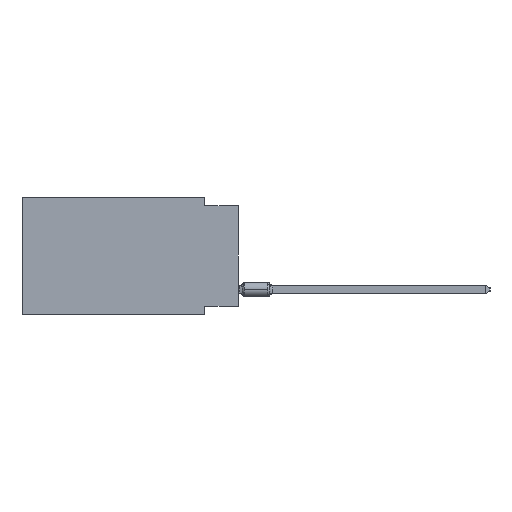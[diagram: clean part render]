
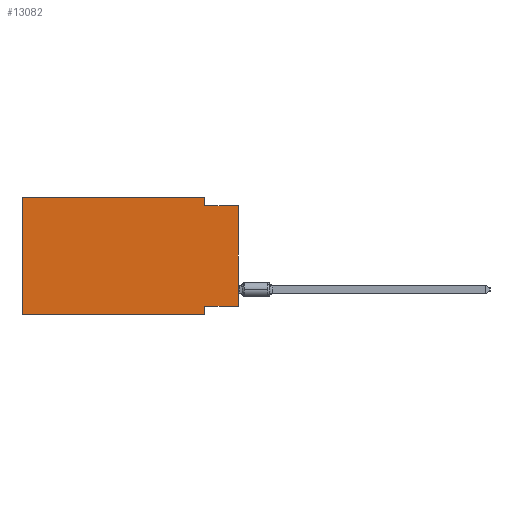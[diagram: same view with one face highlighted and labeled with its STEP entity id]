
A CAD part, left-side view. The second image highlights one B-rep face of the part: STEP entity #13082.
In plain terms, the highlighted planar face has unit normal (-1, 0, 0).
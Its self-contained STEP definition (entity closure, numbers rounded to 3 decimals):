
#56 = CARTESIAN_POINT ( 'NONE',  ( 0., 16.383, 0. ) ) ;
#1926 = LINE ( 'NONE', #31719, #31229 ) ;
#2910 = AXIS2_PLACEMENT_3D ( 'NONE', #56, #14715, #25537 ) ;
#2994 = VERTEX_POINT ( 'NONE', #15073 ) ;
#4694 = EDGE_LOOP ( 'NONE', ( #25086, #36051, #12913, #10213, #41114, #26272, #20955, #39437 ) ) ;
#7222 = VERTEX_POINT ( 'NONE', #24212 ) ;
#7512 = LINE ( 'NONE', #10891, #12361 ) ;
#8205 = VERTEX_POINT ( 'NONE', #41832 ) ;
#8336 = DIRECTION ( 'NONE',  ( 0., 0., -1. ) ) ;
#9957 = VERTEX_POINT ( 'NONE', #23891 ) ;
#10213 = ORIENTED_EDGE ( 'NONE', *, *, #20661, .F. ) ;
#10457 = VERTEX_POINT ( 'NONE', #16375 ) ;
#10891 = CARTESIAN_POINT ( 'NONE',  ( 0., 2.54, 0. ) ) ;
#11546 = EDGE_CURVE ( 'NONE', #20242, #8205, #12090, .T. ) ;
#12041 = EDGE_CURVE ( 'NONE', #31411, #2994, #1926, .T. ) ;
#12090 = LINE ( 'NONE', #23152, #43458 ) ;
#12361 = VECTOR ( 'NONE', #33438, 1000. ) ;
#12913 = ORIENTED_EDGE ( 'NONE', *, *, #18603, .F. ) ;
#13082 = ADVANCED_FACE ( 'NONE', ( #22160 ), #25290, .F. ) ;
#13092 = EDGE_CURVE ( 'NONE', #31411, #15208, #18311, .T. ) ;
#14375 = DIRECTION ( 'NONE',  ( 0., -1., 0. ) ) ;
#14715 = DIRECTION ( 'NONE',  ( 1., 0., 0. ) ) ;
#15073 = CARTESIAN_POINT ( 'NONE',  ( 0., 2.54, -8.89 ) ) ;
#15124 = VECTOR ( 'NONE', #8336, 1000. ) ;
#15208 = VERTEX_POINT ( 'NONE', #45181 ) ;
#16375 = CARTESIAN_POINT ( 'NONE',  ( 0., 2.54, -0.635 ) ) ;
#16580 = DIRECTION ( 'NONE',  ( 0., -1., 0. ) ) ;
#16876 = VECTOR ( 'NONE', #34235, 1000. ) ;
#17485 = EDGE_CURVE ( 'NONE', #10457, #8205, #45370, .T. ) ;
#18311 = LINE ( 'NONE', #22400, #28280 ) ;
#18560 = DIRECTION ( 'NONE',  ( 0., 0., 1. ) ) ;
#18603 = EDGE_CURVE ( 'NONE', #9957, #10457, #7512, .T. ) ;
#20021 = DIRECTION ( 'NONE',  ( 0., 0., 1. ) ) ;
#20242 = VERTEX_POINT ( 'NONE', #43735 ) ;
#20661 = EDGE_CURVE ( 'NONE', #15208, #9957, #37343, .T. ) ;
#20955 = ORIENTED_EDGE ( 'NONE', *, *, #42062, .F. ) ;
#22160 = FACE_OUTER_BOUND ( 'NONE', #4694, .T. ) ;
#22400 = CARTESIAN_POINT ( 'NONE',  ( 0., 16.383, 0. ) ) ;
#23152 = CARTESIAN_POINT ( 'NONE',  ( 0., 0., 0. ) ) ;
#23510 = DIRECTION ( 'NONE',  ( 0., -1., 0. ) ) ;
#23891 = CARTESIAN_POINT ( 'NONE',  ( 0., 2.54, 0. ) ) ;
#24212 = CARTESIAN_POINT ( 'NONE',  ( 0., 2.54, -8.255 ) ) ;
#25086 = ORIENTED_EDGE ( 'NONE', *, *, #11546, .T. ) ;
#25290 = PLANE ( 'NONE',  #2910 ) ;
#25537 = DIRECTION ( 'NONE',  ( 0., 0., -1. ) ) ;
#26272 = ORIENTED_EDGE ( 'NONE', *, *, #12041, .T. ) ;
#26970 = VECTOR ( 'NONE', #14375, 1000. ) ;
#27768 = LINE ( 'NONE', #45751, #16876 ) ;
#28280 = VECTOR ( 'NONE', #18560, 1000. ) ;
#31229 = VECTOR ( 'NONE', #16580, 1000. ) ;
#31411 = VERTEX_POINT ( 'NONE', #39261 ) ;
#31719 = CARTESIAN_POINT ( 'NONE',  ( 0., 16.383, -8.89 ) ) ;
#33438 = DIRECTION ( 'NONE',  ( 0., 0., -1. ) ) ;
#33743 = EDGE_CURVE ( 'NONE', #20242, #7222, #27768, .T. ) ;
#33758 = CARTESIAN_POINT ( 'NONE',  ( 0., 16.383, 0. ) ) ;
#34235 = DIRECTION ( 'NONE',  ( 0., 1., 0. ) ) ;
#36051 = ORIENTED_EDGE ( 'NONE', *, *, #17485, .F. ) ;
#37343 = LINE ( 'NONE', #33758, #26970 ) ;
#38840 = VECTOR ( 'NONE', #23510, 1000. ) ;
#39261 = CARTESIAN_POINT ( 'NONE',  ( 0., 16.383, -8.89 ) ) ;
#39437 = ORIENTED_EDGE ( 'NONE', *, *, #33743, .F. ) ;
#41114 = ORIENTED_EDGE ( 'NONE', *, *, #13092, .F. ) ;
#41237 = CARTESIAN_POINT ( 'NONE',  ( 0., 2.54, -8.89 ) ) ;
#41750 = CARTESIAN_POINT ( 'NONE',  ( 0., 0., -0.635 ) ) ;
#41832 = CARTESIAN_POINT ( 'NONE',  ( 0., 0., -0.635 ) ) ;
#42062 = EDGE_CURVE ( 'NONE', #7222, #2994, #44838, .T. ) ;
#43458 = VECTOR ( 'NONE', #20021, 1000. ) ;
#43735 = CARTESIAN_POINT ( 'NONE',  ( 0., 0., -8.255 ) ) ;
#44838 = LINE ( 'NONE', #41237, #15124 ) ;
#45181 = CARTESIAN_POINT ( 'NONE',  ( 0., 16.383, 0. ) ) ;
#45370 = LINE ( 'NONE', #41750, #38840 ) ;
#45751 = CARTESIAN_POINT ( 'NONE',  ( 0., 0., -8.255 ) ) ;
